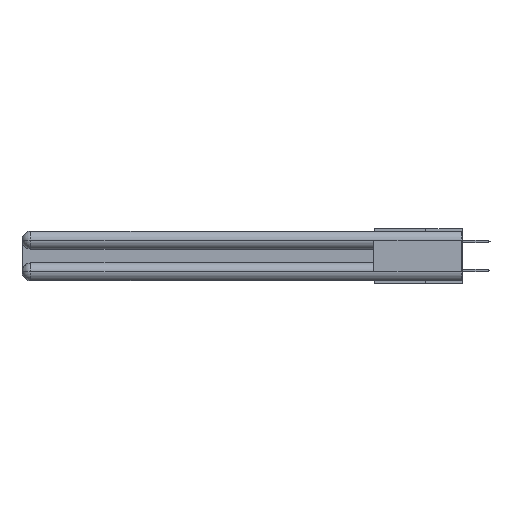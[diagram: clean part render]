
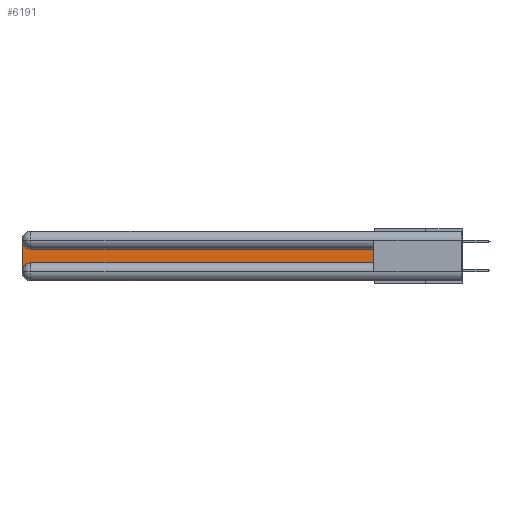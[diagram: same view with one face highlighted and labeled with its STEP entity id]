
A CAD part, left-side view. The second image highlights one B-rep face of the part: STEP entity #6191.
In plain terms, the highlighted planar face has unit normal (-1, 0, 0).
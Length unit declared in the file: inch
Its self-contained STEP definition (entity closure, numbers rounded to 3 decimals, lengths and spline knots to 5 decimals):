
#493 = VERTEX_POINT ( 'NONE', #11407 ) ;
#1187 = LINE ( 'NONE', #26842, #9820 ) ;
#2030 = DIRECTION ( 'NONE',  ( 0., -1., 0. ) ) ;
#3545 = EDGE_CURVE ( 'NONE', #3980, #493, #27556, .T. ) ;
#3980 = VERTEX_POINT ( 'NONE', #23358 ) ;
#4476 = LINE ( 'NONE', #18174, #19440 ) ;
#4901 = VECTOR ( 'NONE', #2030, 39.37008 ) ;
#5016 = DIRECTION ( 'NONE',  ( 0., 0., 1. ) ) ;
#6191 = ADVANCED_FACE ( 'NONE', ( #16038 ), #16096, .F. ) ;
#6534 = AXIS2_PLACEMENT_3D ( 'NONE', #20017, #26457, #7237 ) ;
#6647 = EDGE_CURVE ( 'NONE', #21488, #16920, #25021, .T. ) ;
#7105 = AXIS2_PLACEMENT_3D ( 'NONE', #8772, #19652, #15124 ) ;
#7237 = DIRECTION ( 'NONE',  ( 0., 0., -1. ) ) ;
#7791 = DIRECTION ( 'NONE',  ( 1., 0., 0. ) ) ;
#8686 = EDGE_CURVE ( 'NONE', #16920, #3980, #14958, .T. ) ;
#8772 = CARTESIAN_POINT ( 'NONE',  ( 0.075, 2.94, -0.2775 ) ) ;
#8865 = CARTESIAN_POINT ( 'NONE',  ( 0.075, 3., -0.2175 ) ) ;
#9153 = ORIENTED_EDGE ( 'NONE', *, *, #8686, .T. ) ;
#9820 = VECTOR ( 'NONE', #5016, 39.37008 ) ;
#9968 = EDGE_CURVE ( 'NONE', #493, #21102, #1187, .T. ) ;
#10293 = ORIENTED_EDGE ( 'NONE', *, *, #16790, .T. ) ;
#10340 = CARTESIAN_POINT ( 'NONE',  ( 0.075, 3., -0.0625 ) ) ;
#10781 = EDGE_CURVE ( 'NONE', #21102, #26434, #4476, .T. ) ;
#11407 = CARTESIAN_POINT ( 'NONE',  ( 0.075, 0.6, -0.2175 ) ) ;
#12358 = ORIENTED_EDGE ( 'NONE', *, *, #10781, .T. ) ;
#13044 = ORIENTED_EDGE ( 'NONE', *, *, #6647, .T. ) ;
#13921 = DIRECTION ( 'NONE',  ( 0., 1., 0. ) ) ;
#14958 = CIRCLE ( 'NONE', #7105, 0.06 ) ;
#15124 = DIRECTION ( 'NONE',  ( 0., 0., -1. ) ) ;
#15712 = VECTOR ( 'NONE', #24681, 39.37008 ) ;
#16038 = FACE_OUTER_BOUND ( 'NONE', #26454, .T. ) ;
#16096 = PLANE ( 'NONE',  #19210 ) ;
#16636 = ORIENTED_EDGE ( 'NONE', *, *, #3545, .T. ) ;
#16790 = EDGE_CURVE ( 'NONE', #26434, #21488, #23184, .T. ) ;
#16920 = VERTEX_POINT ( 'NONE', #17821 ) ;
#17821 = CARTESIAN_POINT ( 'NONE',  ( 0.075, 3., -0.2775 ) ) ;
#18174 = CARTESIAN_POINT ( 'NONE',  ( 0.075, 0.6, -0.1225 ) ) ;
#18310 = CARTESIAN_POINT ( 'NONE',  ( 0.075, 2.94, -0.1225 ) ) ;
#18388 = DIRECTION ( 'NONE',  ( 0., 0., -1. ) ) ;
#19210 = AXIS2_PLACEMENT_3D ( 'NONE', #20535, #7791, #18388 ) ;
#19440 = VECTOR ( 'NONE', #13921, 39.37008 ) ;
#19652 = DIRECTION ( 'NONE',  ( 1., 0., 0. ) ) ;
#20017 = CARTESIAN_POINT ( 'NONE',  ( 0.075, 2.94, -0.0625 ) ) ;
#20535 = CARTESIAN_POINT ( 'NONE',  ( 0.075, 3., -0.1225 ) ) ;
#21102 = VERTEX_POINT ( 'NONE', #22775 ) ;
#21488 = VERTEX_POINT ( 'NONE', #10340 ) ;
#22775 = CARTESIAN_POINT ( 'NONE',  ( 0.075, 0.6, -0.1225 ) ) ;
#23184 = CIRCLE ( 'NONE', #6534, 0.06 ) ;
#23358 = CARTESIAN_POINT ( 'NONE',  ( 0.075, 2.94, -0.2175 ) ) ;
#24681 = DIRECTION ( 'NONE',  ( 0., 0., -1. ) ) ;
#25021 = LINE ( 'NONE', #8865, #15712 ) ;
#25792 = CARTESIAN_POINT ( 'NONE',  ( 0.075, 0.6, -0.2175 ) ) ;
#26254 = ORIENTED_EDGE ( 'NONE', *, *, #9968, .T. ) ;
#26434 = VERTEX_POINT ( 'NONE', #18310 ) ;
#26454 = EDGE_LOOP ( 'NONE', ( #12358, #10293, #13044, #9153, #16636, #26254 ) ) ;
#26457 = DIRECTION ( 'NONE',  ( 1., 0., 0. ) ) ;
#26842 = CARTESIAN_POINT ( 'NONE',  ( 0.075, 0.6, -0.2175 ) ) ;
#27556 = LINE ( 'NONE', #25792, #4901 ) ;
